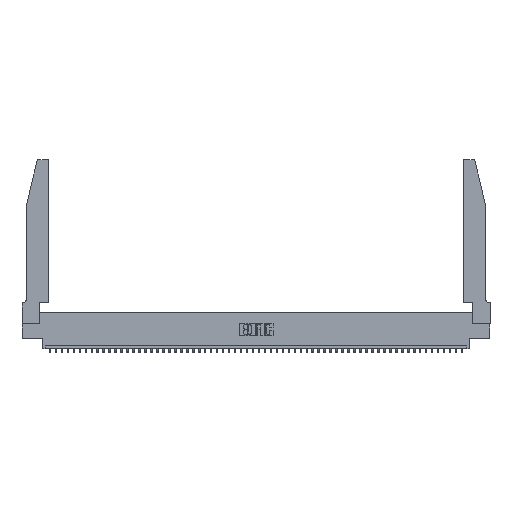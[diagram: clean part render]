
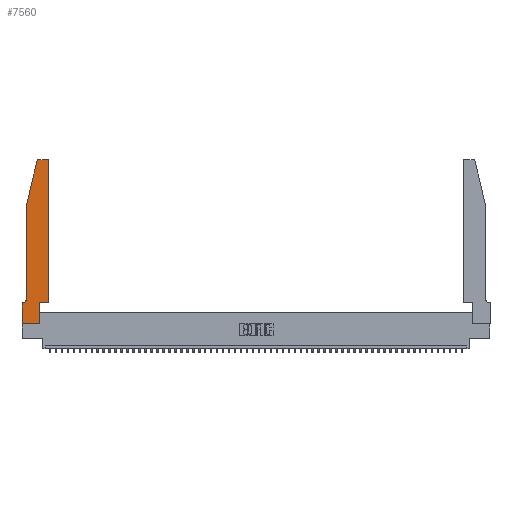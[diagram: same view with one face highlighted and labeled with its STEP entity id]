
A CAD part, top view. The second image highlights one B-rep face of the part: STEP entity #7560.
In plain terms, the highlighted planar face has unit normal (0, 0, 1).
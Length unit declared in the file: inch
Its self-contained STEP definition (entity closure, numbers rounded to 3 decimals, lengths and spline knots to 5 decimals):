
#364 = EDGE_CURVE ( 'NONE', #49684, #29634, #9176, .T. ) ;
#653 = CARTESIAN_POINT ( 'NONE',  ( 0.0055, 0.42, 0.37 ) ) ;
#2025 = CARTESIAN_POINT ( 'NONE',  ( 0.4505, 2.72, 0.37 ) ) ;
#3113 = CARTESIAN_POINT ( 'NONE',  ( 0., 0., 0.37 ) ) ;
#3292 = DIRECTION ( 'NONE',  ( 0., -1., 0. ) ) ;
#3909 = EDGE_CURVE ( 'NONE', #35682, #26759, #10192, .T. ) ;
#4772 = VERTEX_POINT ( 'NONE', #51680 ) ;
#4868 = ORIENTED_EDGE ( 'NONE', *, *, #22232, .T. ) ;
#5364 = VECTOR ( 'NONE', #3292, 39.37008 ) ;
#5461 = LINE ( 'NONE', #32969, #44290 ) ;
#5685 = VERTEX_POINT ( 'NONE', #9339 ) ;
#6014 = ORIENTED_EDGE ( 'NONE', *, *, #42279, .T. ) ;
#6215 = CARTESIAN_POINT ( 'NONE',  ( 0.284, 2.72, 0.37 ) ) ;
#6347 = ORIENTED_EDGE ( 'NONE', *, *, #10399, .T. ) ;
#6348 = DIRECTION ( 'NONE',  ( 0., 0., 1. ) ) ;
#6515 = DIRECTION ( 'NONE',  ( 1., 0., 0. ) ) ;
#7560 = ADVANCED_FACE ( 'NONE', ( #37068 ), #13212, .T. ) ;
#8158 = AXIS2_PLACEMENT_3D ( 'NONE', #17489, #6348, #6515 ) ;
#8430 = VERTEX_POINT ( 'NONE', #41235 ) ;
#8488 = CARTESIAN_POINT ( 'NONE',  ( 0.0755, 0.42, 0.37 ) ) ;
#8689 = CIRCLE ( 'NONE', #23120, 0.03 ) ;
#9006 = EDGE_CURVE ( 'NONE', #8430, #14381, #47152, .T. ) ;
#9176 = LINE ( 'NONE', #39238, #52120 ) ;
#9339 = CARTESIAN_POINT ( 'NONE',  ( 0., 0., 0.37 ) ) ;
#9979 = ORIENTED_EDGE ( 'NONE', *, *, #9006, .T. ) ;
#10192 = LINE ( 'NONE', #50224, #41407 ) ;
#10399 = EDGE_CURVE ( 'NONE', #5685, #4772, #23536, .T. ) ;
#10670 = CARTESIAN_POINT ( 'NONE',  ( 0., 0., 0.37 ) ) ;
#11291 = ORIENTED_EDGE ( 'NONE', *, *, #51807, .T. ) ;
#11340 = CIRCLE ( 'NONE', #14462, 0.03 ) ;
#13212 = PLANE ( 'NONE',  #8158 ) ;
#13897 = DIRECTION ( 'NONE',  ( 1., 0., 0. ) ) ;
#14333 = DIRECTION ( 'NONE',  ( 0., 1., 0. ) ) ;
#14381 = VERTEX_POINT ( 'NONE', #18206 ) ;
#14462 = AXIS2_PLACEMENT_3D ( 'NONE', #6215, #26904, #20157 ) ;
#15444 = CARTESIAN_POINT ( 'NONE',  ( 0.0755, 2., 0.37 ) ) ;
#16623 = DIRECTION ( 'NONE',  ( 0., 0., -1. ) ) ;
#17489 = CARTESIAN_POINT ( 'NONE',  ( 0., 0.35, 0.37 ) ) ;
#17787 = CARTESIAN_POINT ( 'NONE',  ( 0.25487, 2.72718, 0.37 ) ) ;
#17957 = LINE ( 'NONE', #48516, #44089 ) ;
#18206 = CARTESIAN_POINT ( 'NONE',  ( 0., 0.35, 0.37 ) ) ;
#19170 = EDGE_CURVE ( 'NONE', #39111, #49684, #17957, .T. ) ;
#19182 = CARTESIAN_POINT ( 'NONE',  ( 0.2865, 0.35, 0.37 ) ) ;
#19326 = CARTESIAN_POINT ( 'NONE',  ( 0.2605, 2.75, 0.37 ) ) ;
#19445 = VERTEX_POINT ( 'NONE', #40085 ) ;
#20157 = DIRECTION ( 'NONE',  ( 1., 0., 0. ) ) ;
#22232 = EDGE_CURVE ( 'NONE', #19445, #38018, #11340, .T. ) ;
#23120 = AXIS2_PLACEMENT_3D ( 'NONE', #37510, #38010, #46258 ) ;
#23472 = ORIENTED_EDGE ( 'NONE', *, *, #45348, .T. ) ;
#23536 = LINE ( 'NONE', #10670, #50240 ) ;
#23546 = AXIS2_PLACEMENT_3D ( 'NONE', #653, #16623, #49971 ) ;
#25835 = CIRCLE ( 'NONE', #23546, 0.07 ) ;
#26391 = CARTESIAN_POINT ( 'NONE',  ( 0.4205, 2.75, 0.37 ) ) ;
#26759 = VERTEX_POINT ( 'NONE', #8488 ) ;
#26904 = DIRECTION ( 'NONE',  ( 0., 0., 1. ) ) ;
#28617 = CARTESIAN_POINT ( 'NONE',  ( 0.0755, 0.35, 0.37 ) ) ;
#29634 = VERTEX_POINT ( 'NONE', #2025 ) ;
#30564 = DIRECTION ( 'NONE',  ( 1., 0., 0. ) ) ;
#32049 = VECTOR ( 'NONE', #53088, 39.37008 ) ;
#32415 = ORIENTED_EDGE ( 'NONE', *, *, #51941, .T. ) ;
#32803 = VECTOR ( 'NONE', #44693, 39.37008 ) ;
#32870 = ORIENTED_EDGE ( 'NONE', *, *, #47338, .T. ) ;
#32969 = CARTESIAN_POINT ( 'NONE',  ( 0.0755, 2., 0.37 ) ) ;
#33605 = EDGE_CURVE ( 'NONE', #38018, #35682, #5461, .T. ) ;
#33623 = ORIENTED_EDGE ( 'NONE', *, *, #364, .T. ) ;
#34621 = ORIENTED_EDGE ( 'NONE', *, *, #33605, .T. ) ;
#35682 = VERTEX_POINT ( 'NONE', #15444 ) ;
#36333 = VERTEX_POINT ( 'NONE', #26391 ) ;
#37068 = FACE_OUTER_BOUND ( 'NONE', #50852, .T. ) ;
#37336 = CARTESIAN_POINT ( 'NONE',  ( 0.4505, 0.35, 0.37 ) ) ;
#37510 = CARTESIAN_POINT ( 'NONE',  ( 0.4205, 2.72, 0.37 ) ) ;
#37815 = DIRECTION ( 'NONE',  ( 0., -1., 0. ) ) ;
#38010 = DIRECTION ( 'NONE',  ( 0., 0., 1. ) ) ;
#38018 = VERTEX_POINT ( 'NONE', #17787 ) ;
#38299 = VECTOR ( 'NONE', #48499, 39.37008 ) ;
#39111 = VERTEX_POINT ( 'NONE', #40281 ) ;
#39238 = CARTESIAN_POINT ( 'NONE',  ( 0.4505, 0.35, 0.37 ) ) ;
#40085 = CARTESIAN_POINT ( 'NONE',  ( 0.284, 2.75, 0.37 ) ) ;
#40281 = CARTESIAN_POINT ( 'NONE',  ( 0.2865, 0.35, 0.37 ) ) ;
#41135 = LINE ( 'NONE', #3113, #5364 ) ;
#41235 = CARTESIAN_POINT ( 'NONE',  ( 0.0055, 0.35, 0.37 ) ) ;
#41407 = VECTOR ( 'NONE', #37815, 39.37008 ) ;
#41659 = DIRECTION ( 'NONE',  ( -0.239, -0.971, 0. ) ) ;
#42279 = EDGE_CURVE ( 'NONE', #29634, #36333, #8689, .T. ) ;
#43075 = LINE ( 'NONE', #19182, #32049 ) ;
#43993 = ORIENTED_EDGE ( 'NONE', *, *, #3909, .T. ) ;
#44089 = VECTOR ( 'NONE', #13897, 39.37008 ) ;
#44290 = VECTOR ( 'NONE', #41659, 39.37008 ) ;
#44693 = DIRECTION ( 'NONE',  ( -1., 0., 0. ) ) ;
#45348 = EDGE_CURVE ( 'NONE', #26759, #8430, #25835, .T. ) ;
#46258 = DIRECTION ( 'NONE',  ( 1., 0., 0. ) ) ;
#47152 = LINE ( 'NONE', #28617, #32803 ) ;
#47338 = EDGE_CURVE ( 'NONE', #36333, #19445, #50726, .T. ) ;
#48327 = ORIENTED_EDGE ( 'NONE', *, *, #19170, .T. ) ;
#48499 = DIRECTION ( 'NONE',  ( -1., 0., 0. ) ) ;
#48516 = CARTESIAN_POINT ( 'NONE',  ( 0.4505, 0.35, 0.37 ) ) ;
#49684 = VERTEX_POINT ( 'NONE', #37336 ) ;
#49971 = DIRECTION ( 'NONE',  ( -1., 0., 0. ) ) ;
#50224 = CARTESIAN_POINT ( 'NONE',  ( 0.0755, 2., 0.37 ) ) ;
#50240 = VECTOR ( 'NONE', #30564, 39.37008 ) ;
#50726 = LINE ( 'NONE', #19326, #38299 ) ;
#50852 = EDGE_LOOP ( 'NONE', ( #32870, #4868, #34621, #43993, #23472, #9979, #32415, #6347, #11291, #48327, #33623, #6014 ) ) ;
#51680 = CARTESIAN_POINT ( 'NONE',  ( 0.2865, 0., 0.37 ) ) ;
#51807 = EDGE_CURVE ( 'NONE', #4772, #39111, #43075, .T. ) ;
#51941 = EDGE_CURVE ( 'NONE', #14381, #5685, #41135, .T. ) ;
#52120 = VECTOR ( 'NONE', #14333, 39.37008 ) ;
#53088 = DIRECTION ( 'NONE',  ( 0., 1., 0. ) ) ;
